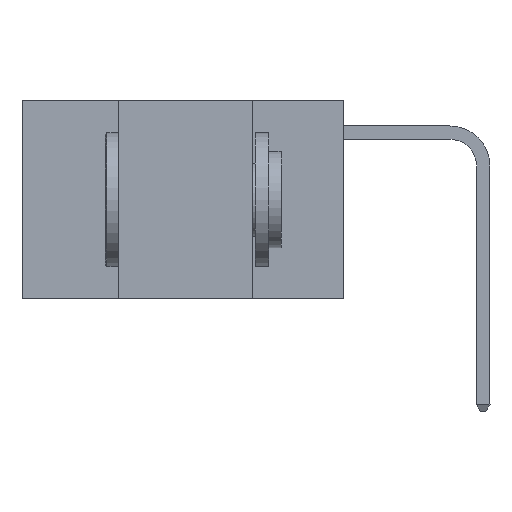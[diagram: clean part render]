
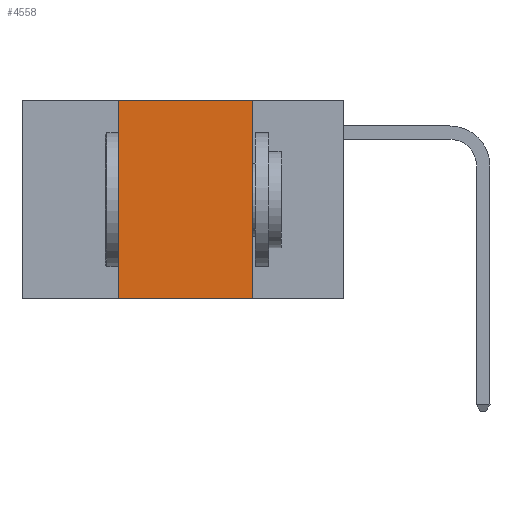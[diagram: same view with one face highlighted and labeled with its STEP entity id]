
A CAD part, left-side view. The second image highlights one B-rep face of the part: STEP entity #4558.
In plain terms, the highlighted planar face has unit normal (-1, 0, 0).
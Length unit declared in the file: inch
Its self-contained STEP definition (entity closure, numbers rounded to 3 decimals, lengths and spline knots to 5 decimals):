
#517 = CARTESIAN_POINT ( 'NONE',  ( 0., 0.17, -0.37 ) ) ;
#540 = CARTESIAN_POINT ( 'NONE',  ( 0., 0.42, 0. ) ) ;
#555 = DIRECTION ( 'NONE',  ( 0., 0., 1. ) ) ;
#1534 = LINE ( 'NONE', #1846, #6356 ) ;
#1570 = VECTOR ( 'NONE', #5573, 39.37008 ) ;
#1574 = LINE ( 'NONE', #5674, #1570 ) ;
#1823 = DIRECTION ( 'NONE',  ( 0., 0., -1. ) ) ;
#1846 = CARTESIAN_POINT ( 'NONE',  ( 0., 0.17, 0. ) ) ;
#1848 = EDGE_CURVE ( 'NONE', #2010, #6093, #1574, .T. ) ;
#2010 = VERTEX_POINT ( 'NONE', #4182 ) ;
#2393 = EDGE_CURVE ( 'NONE', #2010, #5558, #7142, .T. ) ;
#2509 = EDGE_LOOP ( 'NONE', ( #3156, #3169, #3176, #3205 ) ) ;
#3156 = ORIENTED_EDGE ( 'NONE', *, *, #4759, .F. ) ;
#3169 = ORIENTED_EDGE ( 'NONE', *, *, #9556, .F. ) ;
#3176 = ORIENTED_EDGE ( 'NONE', *, *, #2393, .F. ) ;
#3205 = ORIENTED_EDGE ( 'NONE', *, *, #1848, .T. ) ;
#4182 = CARTESIAN_POINT ( 'NONE',  ( 0., 0.42, -0.37 ) ) ;
#4250 = CARTESIAN_POINT ( 'NONE',  ( 0., 0.6, 0. ) ) ;
#4558 = ADVANCED_FACE ( 'NONE', ( #8865 ), #4752, .F. ) ;
#4569 = DIRECTION ( 'NONE',  ( 0., 0., -1. ) ) ;
#4595 = DIRECTION ( 'NONE',  ( 1., 0., 0. ) ) ;
#4616 = CARTESIAN_POINT ( 'NONE',  ( 0., 0.6, 0. ) ) ;
#4752 = PLANE ( 'NONE',  #5617 ) ;
#4759 = EDGE_CURVE ( 'NONE', #7745, #6093, #1534, .T. ) ;
#5558 = VERTEX_POINT ( 'NONE', #6713 ) ;
#5573 = DIRECTION ( 'NONE',  ( 0., -1., 0. ) ) ;
#5617 = AXIS2_PLACEMENT_3D ( 'NONE', #4616, #4595, #4569 ) ;
#5674 = CARTESIAN_POINT ( 'NONE',  ( 0., 0.6, -0.37 ) ) ;
#6093 = VERTEX_POINT ( 'NONE', #517 ) ;
#6356 = VECTOR ( 'NONE', #1823, 39.37008 ) ;
#6713 = CARTESIAN_POINT ( 'NONE',  ( 0., 0.42, 0. ) ) ;
#6965 = VECTOR ( 'NONE', #555, 39.37008 ) ;
#7142 = LINE ( 'NONE', #540, #6965 ) ;
#7505 = DIRECTION ( 'NONE',  ( 0., -1., 0. ) ) ;
#7745 = VERTEX_POINT ( 'NONE', #9134 ) ;
#8865 = FACE_OUTER_BOUND ( 'NONE', #2509, .T. ) ;
#9134 = CARTESIAN_POINT ( 'NONE',  ( 0., 0.17, 0. ) ) ;
#9556 = EDGE_CURVE ( 'NONE', #5558, #7745, #10169, .T. ) ;
#10147 = VECTOR ( 'NONE', #7505, 39.37008 ) ;
#10169 = LINE ( 'NONE', #4250, #10147 ) ;
